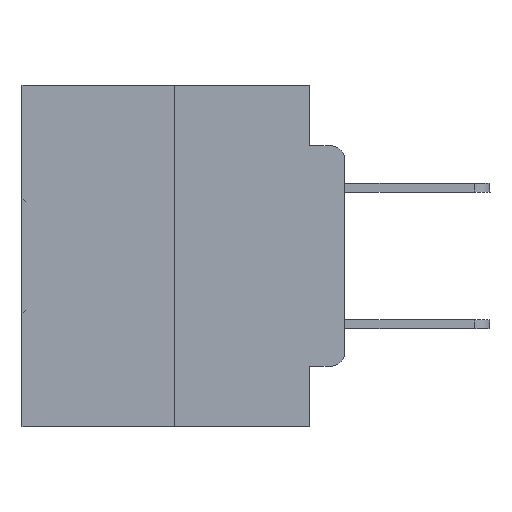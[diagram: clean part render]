
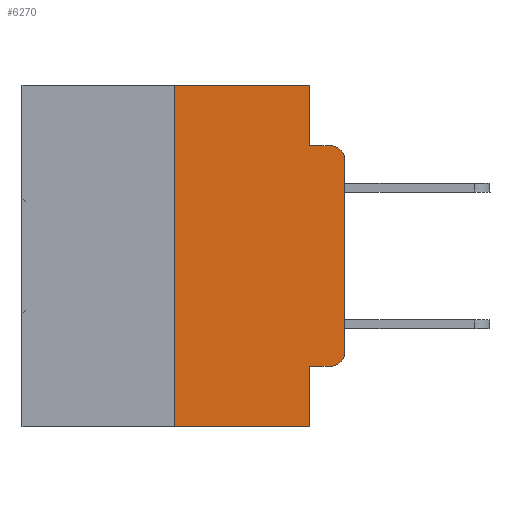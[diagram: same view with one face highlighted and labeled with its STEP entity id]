
A CAD part, left-side view. The second image highlights one B-rep face of the part: STEP entity #6270.
In plain terms, the highlighted planar face has unit normal (-1, 0, 0).
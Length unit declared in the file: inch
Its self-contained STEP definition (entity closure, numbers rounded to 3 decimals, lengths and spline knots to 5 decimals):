
#186 = VECTOR ( 'NONE', #27132, 39.37008 ) ;
#645 = ORIENTED_EDGE ( 'NONE', *, *, #1928, .T. ) ;
#689 = CARTESIAN_POINT ( 'NONE',  ( 0., 0., -0.1085 ) ) ;
#782 = ORIENTED_EDGE ( 'NONE', *, *, #25230, .F. ) ;
#910 = LINE ( 'NONE', #12027, #25774 ) ;
#1137 = VERTEX_POINT ( 'NONE', #6403 ) ;
#1277 = CARTESIAN_POINT ( 'NONE',  ( 0., 0.051, -0.0885 ) ) ;
#1399 = CARTESIAN_POINT ( 'NONE',  ( 0., 0.473, -0.5 ) ) ;
#1459 = VECTOR ( 'NONE', #17092, 39.37008 ) ;
#1928 = EDGE_CURVE ( 'NONE', #15741, #15480, #6120, .T. ) ;
#1938 = LINE ( 'NONE', #1277, #20791 ) ;
#2416 = CARTESIAN_POINT ( 'NONE',  ( 0., 0.02, -0.1085 ) ) ;
#3227 = LINE ( 'NONE', #29330, #32487 ) ;
#3274 = DIRECTION ( 'NONE',  ( 0., 0., -1. ) ) ;
#3494 = CARTESIAN_POINT ( 'NONE',  ( 0., 0.473, 0. ) ) ;
#3771 = ORIENTED_EDGE ( 'NONE', *, *, #29297, .F. ) ;
#4181 = DIRECTION ( 'NONE',  ( 0., 0., 1. ) ) ;
#4451 = VERTEX_POINT ( 'NONE', #25589 ) ;
#4965 = DIRECTION ( 'NONE',  ( -1., 0., 0. ) ) ;
#4994 = EDGE_CURVE ( 'NONE', #4451, #19190, #22797, .T. ) ;
#5316 = ORIENTED_EDGE ( 'NONE', *, *, #31831, .T. ) ;
#5908 = CIRCLE ( 'NONE', #26873, 0.02 ) ;
#6120 = CIRCLE ( 'NONE', #19500, 0.02 ) ;
#6240 = DIRECTION ( 'NONE',  ( 0., -1., 0. ) ) ;
#6270 = ADVANCED_FACE ( 'NONE', ( #14363 ), #21223, .F. ) ;
#6347 = VECTOR ( 'NONE', #19133, 39.37008 ) ;
#6403 = CARTESIAN_POINT ( 'NONE',  ( 0., 0.25, 0. ) ) ;
#6661 = CARTESIAN_POINT ( 'NONE',  ( 0., 0.02, -0.3915 ) ) ;
#6682 = CARTESIAN_POINT ( 'NONE',  ( 0., 0.051, -0.0885 ) ) ;
#6818 = LINE ( 'NONE', #30716, #18082 ) ;
#6950 = EDGE_CURVE ( 'NONE', #26391, #23656, #1938, .T. ) ;
#7139 = CARTESIAN_POINT ( 'NONE',  ( 0., 0.02, -0.0885 ) ) ;
#7343 = VERTEX_POINT ( 'NONE', #689 ) ;
#9077 = VECTOR ( 'NONE', #25798, 39.37008 ) ;
#9789 = EDGE_CURVE ( 'NONE', #12051, #19190, #33009, .T. ) ;
#9885 = LINE ( 'NONE', #19769, #1459 ) ;
#10352 = DIRECTION ( 'NONE',  ( 0., -1., 0. ) ) ;
#11891 = EDGE_CURVE ( 'NONE', #1137, #21553, #6818, .T. ) ;
#12027 = CARTESIAN_POINT ( 'NONE',  ( 0., 0., 0. ) ) ;
#12051 = VERTEX_POINT ( 'NONE', #31502 ) ;
#12629 = DIRECTION ( 'NONE',  ( 0., 0., -1. ) ) ;
#14184 = ORIENTED_EDGE ( 'NONE', *, *, #4994, .T. ) ;
#14363 = FACE_OUTER_BOUND ( 'NONE', #19380, .T. ) ;
#15480 = VERTEX_POINT ( 'NONE', #30289 ) ;
#15548 = LINE ( 'NONE', #16741, #9077 ) ;
#15741 = VERTEX_POINT ( 'NONE', #29847 ) ;
#16398 = DIRECTION ( 'NONE',  ( 1., 0., 0. ) ) ;
#16490 = ORIENTED_EDGE ( 'NONE', *, *, #9789, .F. ) ;
#16741 = CARTESIAN_POINT ( 'NONE',  ( 0., 0.25, 0. ) ) ;
#17013 = DIRECTION ( 'NONE',  ( -1., 0., 0. ) ) ;
#17092 = DIRECTION ( 'NONE',  ( 0., 0., -1. ) ) ;
#18034 = ORIENTED_EDGE ( 'NONE', *, *, #11891, .F. ) ;
#18082 = VECTOR ( 'NONE', #10352, 39.37008 ) ;
#18745 = ORIENTED_EDGE ( 'NONE', *, *, #28682, .T. ) ;
#19132 = DIRECTION ( 'NONE',  ( 0., -1., 0. ) ) ;
#19133 = DIRECTION ( 'NONE',  ( 0., -1., 0. ) ) ;
#19190 = VERTEX_POINT ( 'NONE', #24478 ) ;
#19380 = EDGE_LOOP ( 'NONE', ( #5316, #18745, #25427, #3771, #18034, #782, #14184, #16490, #20571, #645 ) ) ;
#19500 = AXIS2_PLACEMENT_3D ( 'NONE', #6661, #17013, #19590 ) ;
#19590 = DIRECTION ( 'NONE',  ( 0., 0., -1. ) ) ;
#19769 = CARTESIAN_POINT ( 'NONE',  ( 0., 0.051, 0. ) ) ;
#20571 = ORIENTED_EDGE ( 'NONE', *, *, #26392, .T. ) ;
#20791 = VECTOR ( 'NONE', #19132, 39.37008 ) ;
#20874 = AXIS2_PLACEMENT_3D ( 'NONE', #3494, #16398, #3274 ) ;
#21223 = PLANE ( 'NONE',  #20874 ) ;
#21553 = VERTEX_POINT ( 'NONE', #29382 ) ;
#22797 = LINE ( 'NONE', #1399, #6347 ) ;
#23656 = VERTEX_POINT ( 'NONE', #7139 ) ;
#24478 = CARTESIAN_POINT ( 'NONE',  ( 0., 0.051, -0.5 ) ) ;
#25230 = EDGE_CURVE ( 'NONE', #4451, #1137, #15548, .T. ) ;
#25427 = ORIENTED_EDGE ( 'NONE', *, *, #6950, .F. ) ;
#25589 = CARTESIAN_POINT ( 'NONE',  ( 0., 0.25, -0.5 ) ) ;
#25774 = VECTOR ( 'NONE', #4181, 39.37008 ) ;
#25798 = DIRECTION ( 'NONE',  ( 0., 0., 1. ) ) ;
#26391 = VERTEX_POINT ( 'NONE', #6682 ) ;
#26392 = EDGE_CURVE ( 'NONE', #12051, #15741, #3227, .T. ) ;
#26873 = AXIS2_PLACEMENT_3D ( 'NONE', #2416, #4965, #12629 ) ;
#27132 = DIRECTION ( 'NONE',  ( 0., 0., -1. ) ) ;
#28682 = EDGE_CURVE ( 'NONE', #7343, #23656, #5908, .T. ) ;
#29297 = EDGE_CURVE ( 'NONE', #21553, #26391, #9885, .T. ) ;
#29330 = CARTESIAN_POINT ( 'NONE',  ( 0., 0.051, -0.4115 ) ) ;
#29355 = CARTESIAN_POINT ( 'NONE',  ( 0., 0.051, 0. ) ) ;
#29382 = CARTESIAN_POINT ( 'NONE',  ( 0., 0.051, 0. ) ) ;
#29847 = CARTESIAN_POINT ( 'NONE',  ( 0., 0.02, -0.4115 ) ) ;
#30289 = CARTESIAN_POINT ( 'NONE',  ( 0., 0., -0.3915 ) ) ;
#30716 = CARTESIAN_POINT ( 'NONE',  ( 0., 0.473, 0. ) ) ;
#31502 = CARTESIAN_POINT ( 'NONE',  ( 0., 0.051, -0.4115 ) ) ;
#31831 = EDGE_CURVE ( 'NONE', #15480, #7343, #910, .T. ) ;
#32487 = VECTOR ( 'NONE', #6240, 39.37008 ) ;
#33009 = LINE ( 'NONE', #29355, #186 ) ;
